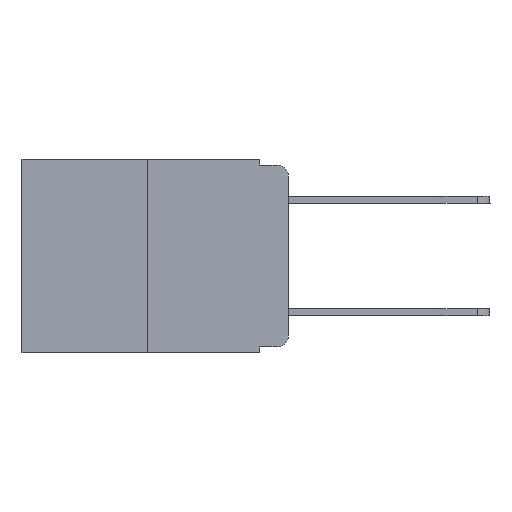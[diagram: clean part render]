
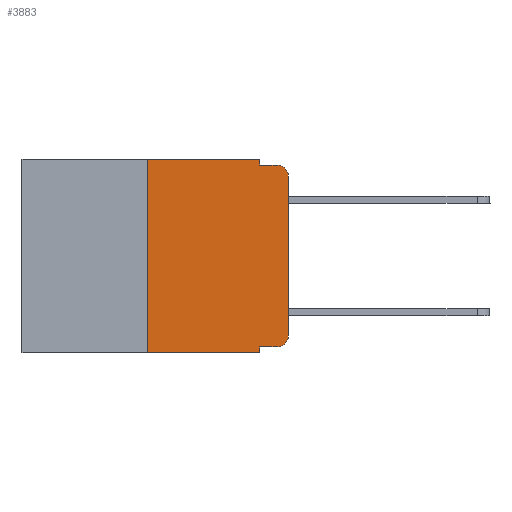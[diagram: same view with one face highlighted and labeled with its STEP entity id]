
A CAD part, left-side view. The second image highlights one B-rep face of the part: STEP entity #3883.
In plain terms, the highlighted planar face has unit normal (-1, 0, 0).
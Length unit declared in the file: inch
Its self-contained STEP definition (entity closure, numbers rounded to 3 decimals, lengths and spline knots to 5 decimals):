
#96 = CARTESIAN_POINT ( 'NONE',  ( 0., 0.25, 0. ) ) ;
#99 = ORIENTED_EDGE ( 'NONE', *, *, #8988, .F. ) ;
#291 = CARTESIAN_POINT ( 'NONE',  ( 0., 0., 0. ) ) ;
#467 = VERTEX_POINT ( 'NONE', #6819 ) ;
#609 = CARTESIAN_POINT ( 'NONE',  ( 0., 0., -0.03 ) ) ;
#866 = DIRECTION ( 'NONE',  ( 0., 0., 1. ) ) ;
#908 = CARTESIAN_POINT ( 'NONE',  ( 0., 0.051, -0.343 ) ) ;
#916 = ORIENTED_EDGE ( 'NONE', *, *, #5197, .F. ) ;
#969 = VECTOR ( 'NONE', #8826, 39.37008 ) ;
#1095 = CARTESIAN_POINT ( 'NONE',  ( 0., 0.02, -0.313 ) ) ;
#1553 = VECTOR ( 'NONE', #1571, 39.37008 ) ;
#1571 = DIRECTION ( 'NONE',  ( 0., -1., 0. ) ) ;
#2039 = VERTEX_POINT ( 'NONE', #2925 ) ;
#2081 = ORIENTED_EDGE ( 'NONE', *, *, #6801, .T. ) ;
#2128 = VERTEX_POINT ( 'NONE', #96 ) ;
#2388 = VERTEX_POINT ( 'NONE', #609 ) ;
#2393 = AXIS2_PLACEMENT_3D ( 'NONE', #4944, #5704, #7214 ) ;
#2415 = CARTESIAN_POINT ( 'NONE',  ( 0., 0.051, 0. ) ) ;
#2742 = VECTOR ( 'NONE', #8341, 39.37008 ) ;
#2826 = CARTESIAN_POINT ( 'NONE',  ( 0., 0.051, -0.01 ) ) ;
#2869 = AXIS2_PLACEMENT_3D ( 'NONE', #3492, #5064, #5764 ) ;
#2874 = FACE_OUTER_BOUND ( 'NONE', #6219, .T. ) ;
#2925 = CARTESIAN_POINT ( 'NONE',  ( 0., 0.051, -0.01 ) ) ;
#2937 = VERTEX_POINT ( 'NONE', #3933 ) ;
#2980 = CARTESIAN_POINT ( 'NONE',  ( 0., 0.02, -0.333 ) ) ;
#3008 = LINE ( 'NONE', #5613, #6884 ) ;
#3032 = CARTESIAN_POINT ( 'NONE',  ( 0., 0.473, -0.343 ) ) ;
#3234 = ORIENTED_EDGE ( 'NONE', *, *, #4645, .F. ) ;
#3255 = EDGE_CURVE ( 'NONE', #467, #4339, #7109, .T. ) ;
#3463 = PLANE ( 'NONE',  #2393 ) ;
#3492 = CARTESIAN_POINT ( 'NONE',  ( 0., 0.02, -0.03 ) ) ;
#3515 = ORIENTED_EDGE ( 'NONE', *, *, #9091, .T. ) ;
#3569 = LINE ( 'NONE', #3032, #1553 ) ;
#3731 = CIRCLE ( 'NONE', #2869, 0.02 ) ;
#3883 = ADVANCED_FACE ( 'NONE', ( #2874 ), #3463, .F. ) ;
#3933 = CARTESIAN_POINT ( 'NONE',  ( 0., 0.25, -0.343 ) ) ;
#4260 = VECTOR ( 'NONE', #866, 39.37008 ) ;
#4339 = VERTEX_POINT ( 'NONE', #2980 ) ;
#4382 = LINE ( 'NONE', #9130, #4260 ) ;
#4456 = VERTEX_POINT ( 'NONE', #2415 ) ;
#4645 = EDGE_CURVE ( 'NONE', #2039, #5273, #6152, .T. ) ;
#4777 = VECTOR ( 'NONE', #5987, 39.37008 ) ;
#4883 = EDGE_CURVE ( 'NONE', #4339, #7045, #9192, .T. ) ;
#4944 = CARTESIAN_POINT ( 'NONE',  ( 0., 0.473, 0. ) ) ;
#4968 = EDGE_CURVE ( 'NONE', #7045, #2388, #6144, .T. ) ;
#5064 = DIRECTION ( 'NONE',  ( -1., 0., 0. ) ) ;
#5085 = CARTESIAN_POINT ( 'NONE',  ( 0., 0.051, -0.333 ) ) ;
#5197 = EDGE_CURVE ( 'NONE', #2937, #2128, #4382, .T. ) ;
#5273 = VERTEX_POINT ( 'NONE', #6058 ) ;
#5336 = CARTESIAN_POINT ( 'NONE',  ( 0., 0.051, 0. ) ) ;
#5446 = VECTOR ( 'NONE', #6321, 39.37008 ) ;
#5613 = CARTESIAN_POINT ( 'NONE',  ( 0., 0.051, 0. ) ) ;
#5704 = DIRECTION ( 'NONE',  ( 1., 0., 0. ) ) ;
#5764 = DIRECTION ( 'NONE',  ( 0., 0., -1. ) ) ;
#5987 = DIRECTION ( 'NONE',  ( 0., -1., 0. ) ) ;
#6058 = CARTESIAN_POINT ( 'NONE',  ( 0., 0.02, -0.01 ) ) ;
#6144 = LINE ( 'NONE', #291, #5446 ) ;
#6152 = LINE ( 'NONE', #2826, #8968 ) ;
#6219 = EDGE_LOOP ( 'NONE', ( #6919, #2081, #3234, #6858, #6738, #916, #3515, #99, #6622, #7505 ) ) ;
#6321 = DIRECTION ( 'NONE',  ( 0., 0., 1. ) ) ;
#6372 = DIRECTION ( 'NONE',  ( -1., 0., 0. ) ) ;
#6384 = DIRECTION ( 'NONE',  ( 0., 0., -1. ) ) ;
#6572 = AXIS2_PLACEMENT_3D ( 'NONE', #1095, #6372, #7135 ) ;
#6622 = ORIENTED_EDGE ( 'NONE', *, *, #3255, .T. ) ;
#6738 = ORIENTED_EDGE ( 'NONE', *, *, #6921, .F. ) ;
#6801 = EDGE_CURVE ( 'NONE', #2388, #5273, #3731, .T. ) ;
#6819 = CARTESIAN_POINT ( 'NONE',  ( 0., 0.051, -0.333 ) ) ;
#6858 = ORIENTED_EDGE ( 'NONE', *, *, #9707, .F. ) ;
#6884 = VECTOR ( 'NONE', #6384, 39.37008 ) ;
#6919 = ORIENTED_EDGE ( 'NONE', *, *, #4968, .T. ) ;
#6921 = EDGE_CURVE ( 'NONE', #2128, #4456, #7257, .T. ) ;
#7045 = VERTEX_POINT ( 'NONE', #9222 ) ;
#7109 = LINE ( 'NONE', #5085, #969 ) ;
#7135 = DIRECTION ( 'NONE',  ( 0., 0., -1. ) ) ;
#7214 = DIRECTION ( 'NONE',  ( 0., 0., -1. ) ) ;
#7257 = LINE ( 'NONE', #8875, #4777 ) ;
#7505 = ORIENTED_EDGE ( 'NONE', *, *, #4883, .T. ) ;
#8101 = DIRECTION ( 'NONE',  ( 0., -1., 0. ) ) ;
#8341 = DIRECTION ( 'NONE',  ( 0., 0., -1. ) ) ;
#8826 = DIRECTION ( 'NONE',  ( 0., -1., 0. ) ) ;
#8875 = CARTESIAN_POINT ( 'NONE',  ( 0., 0.473, 0. ) ) ;
#8968 = VECTOR ( 'NONE', #8101, 39.37008 ) ;
#8988 = EDGE_CURVE ( 'NONE', #467, #9456, #9087, .T. ) ;
#9087 = LINE ( 'NONE', #5336, #2742 ) ;
#9091 = EDGE_CURVE ( 'NONE', #2937, #9456, #3569, .T. ) ;
#9130 = CARTESIAN_POINT ( 'NONE',  ( 0., 0.25, 0. ) ) ;
#9192 = CIRCLE ( 'NONE', #6572, 0.02 ) ;
#9222 = CARTESIAN_POINT ( 'NONE',  ( 0., 0., -0.313 ) ) ;
#9456 = VERTEX_POINT ( 'NONE', #908 ) ;
#9707 = EDGE_CURVE ( 'NONE', #4456, #2039, #3008, .T. ) ;
